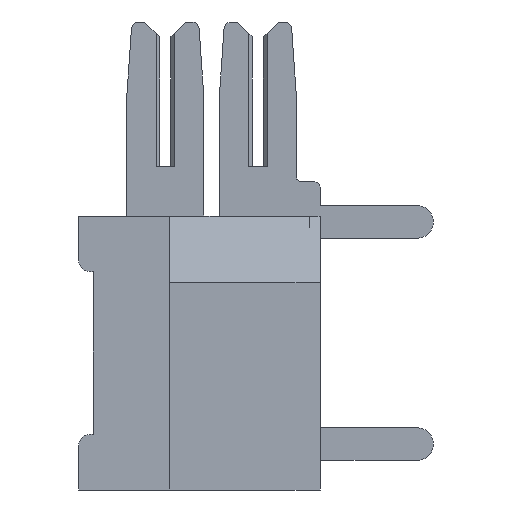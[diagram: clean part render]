
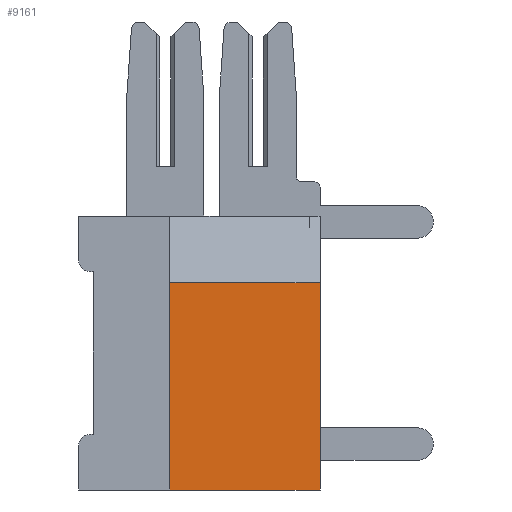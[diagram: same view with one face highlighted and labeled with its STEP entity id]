
A CAD part, left-side view. The second image highlights one B-rep face of the part: STEP entity #9161.
In plain terms, the highlighted planar face has unit normal (-1, 0, 0).
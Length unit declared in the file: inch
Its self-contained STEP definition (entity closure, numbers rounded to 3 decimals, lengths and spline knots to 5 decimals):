
#992 = CARTESIAN_POINT ( 'NONE',  ( 0., 0.203, -0.37 ) ) ;
#1117 = VERTEX_POINT ( 'NONE', #2922 ) ;
#1138 = DIRECTION ( 'NONE',  ( 0., 1., 0. ) ) ;
#1271 = ORIENTED_EDGE ( 'NONE', *, *, #7492, .F. ) ;
#1460 = ORIENTED_EDGE ( 'NONE', *, *, #10384, .T. ) ;
#1510 = VERTEX_POINT ( 'NONE', #5671 ) ;
#1666 = VECTOR ( 'NONE', #1138, 39.37008 ) ;
#1877 = CARTESIAN_POINT ( 'NONE',  ( 0., 0., -0.37 ) ) ;
#2039 = EDGE_CURVE ( 'NONE', #9396, #1117, #5213, .T. ) ;
#2575 = CARTESIAN_POINT ( 'NONE',  ( 0., 0.326, 0. ) ) ;
#2922 = CARTESIAN_POINT ( 'NONE',  ( 0., 0., -0.09 ) ) ;
#2979 = CARTESIAN_POINT ( 'NONE',  ( 0., 0., -0.09 ) ) ;
#3412 = CARTESIAN_POINT ( 'NONE',  ( 0., 0.326, -0.37 ) ) ;
#3604 = ORIENTED_EDGE ( 'NONE', *, *, #2039, .T. ) ;
#3680 = DIRECTION ( 'NONE',  ( 0., 0., 1. ) ) ;
#3750 = VECTOR ( 'NONE', #7738, 39.37008 ) ;
#3977 = VECTOR ( 'NONE', #3680, 39.37008 ) ;
#4533 = DIRECTION ( 'NONE',  ( 0., 0., 1. ) ) ;
#5213 = LINE ( 'NONE', #7128, #8521 ) ;
#5671 = CARTESIAN_POINT ( 'NONE',  ( 0., 0.203, -0.09 ) ) ;
#6052 = PLANE ( 'NONE',  #9762 ) ;
#6156 = ORIENTED_EDGE ( 'NONE', *, *, #8765, .T. ) ;
#6974 = DIRECTION ( 'NONE',  ( 0., 0., -1. ) ) ;
#7128 = CARTESIAN_POINT ( 'NONE',  ( 0., 0., 0. ) ) ;
#7492 = EDGE_CURVE ( 'NONE', #8268, #1510, #11262, .T. ) ;
#7738 = DIRECTION ( 'NONE',  ( 0., -1., 0. ) ) ;
#7887 = FACE_OUTER_BOUND ( 'NONE', #7888, .T. ) ;
#7888 = EDGE_LOOP ( 'NONE', ( #3604, #6156, #1271, #1460 ) ) ;
#8134 = LINE ( 'NONE', #3412, #3750 ) ;
#8268 = VERTEX_POINT ( 'NONE', #992 ) ;
#8521 = VECTOR ( 'NONE', #4533, 39.37008 ) ;
#8743 = DIRECTION ( 'NONE',  ( 1., 0., 0. ) ) ;
#8765 = EDGE_CURVE ( 'NONE', #1117, #1510, #11120, .T. ) ;
#8931 = CARTESIAN_POINT ( 'NONE',  ( 0., 0.203, -0.37 ) ) ;
#9161 = ADVANCED_FACE ( 'NONE', ( #7887 ), #6052, .F. ) ;
#9396 = VERTEX_POINT ( 'NONE', #1877 ) ;
#9762 = AXIS2_PLACEMENT_3D ( 'NONE', #2575, #8743, #6974 ) ;
#10384 = EDGE_CURVE ( 'NONE', #8268, #9396, #8134, .T. ) ;
#11120 = LINE ( 'NONE', #2979, #1666 ) ;
#11262 = LINE ( 'NONE', #8931, #3977 ) ;
